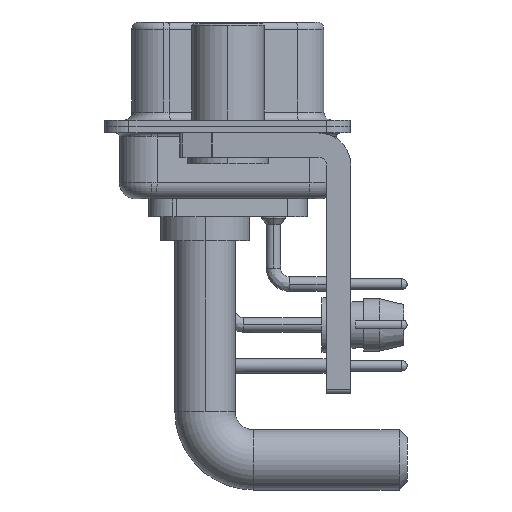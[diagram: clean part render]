
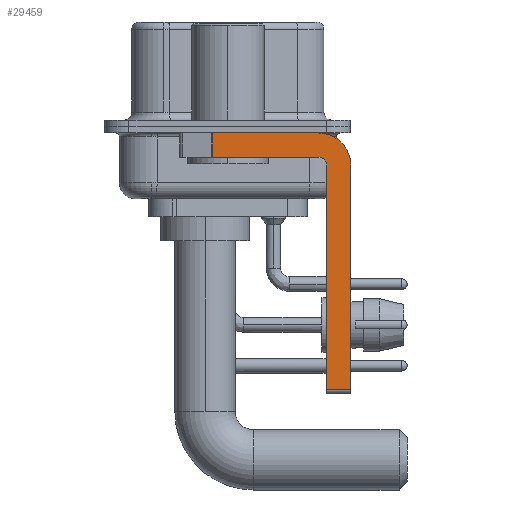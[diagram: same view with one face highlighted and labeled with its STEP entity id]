
A CAD part, left-side view. The second image highlights one B-rep face of the part: STEP entity #29459.
In plain terms, the highlighted planar face has unit normal (-1, 0, 0).
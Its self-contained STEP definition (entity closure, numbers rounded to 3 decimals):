
#224 = LINE ( 'NONE', #23888, #13601 ) ;
#378 = CARTESIAN_POINT ( 'NONE',  ( -2.9, 0.978, -1.9 ) ) ;
#510 = CARTESIAN_POINT ( 'NONE',  ( -2.9, -6.15, -2.4 ) ) ;
#787 = VECTOR ( 'NONE', #9765, 1000. ) ;
#1475 = CARTESIAN_POINT ( 'NONE',  ( -2.9, 3., -0.4 ) ) ;
#1521 = CARTESIAN_POINT ( 'NONE',  ( -2.9, -5.65, -1.9 ) ) ;
#1759 = PLANE ( 'NONE',  #33223 ) ;
#2464 = AXIS2_PLACEMENT_3D ( 'NONE', #25085, #10362, #7445 ) ;
#3238 = EDGE_CURVE ( 'NONE', #21396, #4226, #224, .T. ) ;
#3777 = VERTEX_POINT ( 'NONE', #33360 ) ;
#4226 = VERTEX_POINT ( 'NONE', #21986 ) ;
#5029 = CARTESIAN_POINT ( 'NONE',  ( -2.9, 0.978, -1.9 ) ) ;
#5173 = ORIENTED_EDGE ( 'NONE', *, *, #12364, .T. ) ;
#6226 = VERTEX_POINT ( 'NONE', #16665 ) ;
#6726 = AXIS2_PLACEMENT_3D ( 'NONE', #36991, #19509, #25343 ) ;
#7445 = DIRECTION ( 'NONE',  ( 0., 0., -1. ) ) ;
#7468 = LINE ( 'NONE', #14063, #7837 ) ;
#7837 = VECTOR ( 'NONE', #10576, 1000. ) ;
#9112 = LINE ( 'NONE', #21125, #31319 ) ;
#9602 = CARTESIAN_POINT ( 'NONE',  ( -2.9, -5.65, -0.4 ) ) ;
#9765 = DIRECTION ( 'NONE',  ( 0., 0., -1. ) ) ;
#10032 = DIRECTION ( 'NONE',  ( 0., -1., 0. ) ) ;
#10362 = DIRECTION ( 'NONE',  ( 1., 0., 0. ) ) ;
#10441 = VECTOR ( 'NONE', #10032, 1000. ) ;
#10576 = DIRECTION ( 'NONE',  ( 0., 0., 1. ) ) ;
#10686 = CARTESIAN_POINT ( 'NONE',  ( -2.9, -5.65, -2.4 ) ) ;
#12364 = EDGE_CURVE ( 'NONE', #3777, #31054, #31613, .T. ) ;
#12826 = FACE_OUTER_BOUND ( 'NONE', #35454, .T. ) ;
#13601 = VECTOR ( 'NONE', #30875, 1000. ) ;
#13970 = ORIENTED_EDGE ( 'NONE', *, *, #27998, .F. ) ;
#14063 = CARTESIAN_POINT ( 'NONE',  ( -2.9, -6.15, -16.6 ) ) ;
#15547 = CARTESIAN_POINT ( 'NONE',  ( -2.9, -6.15, -16.35 ) ) ;
#15851 = LINE ( 'NONE', #1475, #10441 ) ;
#16665 = CARTESIAN_POINT ( 'NONE',  ( -2.9, -5.65, -1.9 ) ) ;
#16918 = CARTESIAN_POINT ( 'NONE',  ( -2.9, -7.65, -2.4 ) ) ;
#18349 = ORIENTED_EDGE ( 'NONE', *, *, #24540, .F. ) ;
#18546 = EDGE_CURVE ( 'NONE', #23027, #4226, #9112, .T. ) ;
#18634 = ORIENTED_EDGE ( 'NONE', *, *, #31672, .F. ) ;
#19509 = DIRECTION ( 'NONE',  ( -1., 0., 0. ) ) ;
#20940 = DIRECTION ( 'NONE',  ( 0., -1., 0. ) ) ;
#21125 = CARTESIAN_POINT ( 'NONE',  ( -2.9, -5.65, -16.35 ) ) ;
#21396 = VERTEX_POINT ( 'NONE', #16918 ) ;
#21986 = CARTESIAN_POINT ( 'NONE',  ( -2.9, -7.65, -16.35 ) ) ;
#23027 = VERTEX_POINT ( 'NONE', #15547 ) ;
#23307 = ORIENTED_EDGE ( 'NONE', *, *, #31693, .F. ) ;
#23888 = CARTESIAN_POINT ( 'NONE',  ( -2.9, -7.65, -2.4 ) ) ;
#24319 = ORIENTED_EDGE ( 'NONE', *, *, #29860, .F. ) ;
#24540 = EDGE_CURVE ( 'NONE', #25263, #21396, #27260, .T. ) ;
#24649 = DIRECTION ( 'NONE',  ( 1., 0., 0. ) ) ;
#25085 = CARTESIAN_POINT ( 'NONE',  ( -2.9, -5.65, -2.4 ) ) ;
#25263 = VERTEX_POINT ( 'NONE', #9602 ) ;
#25343 = DIRECTION ( 'NONE',  ( 0., 0., 1. ) ) ;
#27260 = CIRCLE ( 'NONE', #2464, 2. ) ;
#27730 = DIRECTION ( 'NONE',  ( 0., 1., 0. ) ) ;
#27798 = CIRCLE ( 'NONE', #6726, 0.5 ) ;
#27998 = EDGE_CURVE ( 'NONE', #23027, #34364, #7468, .T. ) ;
#28918 = VECTOR ( 'NONE', #27730, 1000. ) ;
#29459 = ADVANCED_FACE ( 'NONE', ( #12826 ), #1759, .F. ) ;
#29860 = EDGE_CURVE ( 'NONE', #6226, #31054, #30629, .T. ) ;
#30357 = ORIENTED_EDGE ( 'NONE', *, *, #3238, .F. ) ;
#30629 = LINE ( 'NONE', #1521, #28918 ) ;
#30875 = DIRECTION ( 'NONE',  ( 0., 0., -1. ) ) ;
#31054 = VERTEX_POINT ( 'NONE', #378 ) ;
#31319 = VECTOR ( 'NONE', #20940, 1000. ) ;
#31613 = LINE ( 'NONE', #5029, #787 ) ;
#31672 = EDGE_CURVE ( 'NONE', #3777, #25263, #15851, .T. ) ;
#31693 = EDGE_CURVE ( 'NONE', #34364, #6226, #27798, .T. ) ;
#33223 = AXIS2_PLACEMENT_3D ( 'NONE', #10686, #24649, #34352 ) ;
#33360 = CARTESIAN_POINT ( 'NONE',  ( -2.9, 0.978, -0.4 ) ) ;
#34352 = DIRECTION ( 'NONE',  ( 0., 0., -1. ) ) ;
#34364 = VERTEX_POINT ( 'NONE', #510 ) ;
#35454 = EDGE_LOOP ( 'NONE', ( #18634, #5173, #24319, #23307, #13970, #36332, #30357, #18349 ) ) ;
#36332 = ORIENTED_EDGE ( 'NONE', *, *, #18546, .T. ) ;
#36991 = CARTESIAN_POINT ( 'NONE',  ( -2.9, -5.65, -2.4 ) ) ;
